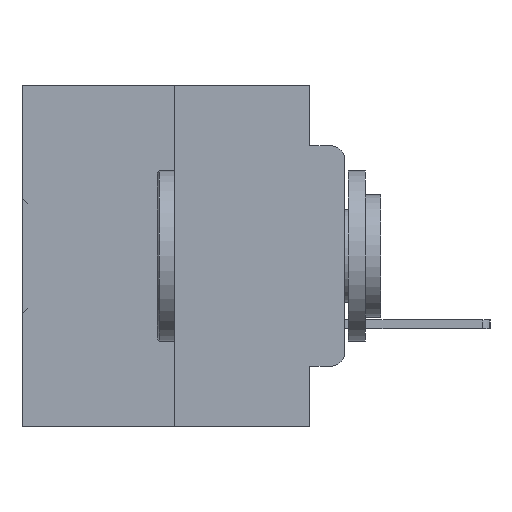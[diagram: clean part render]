
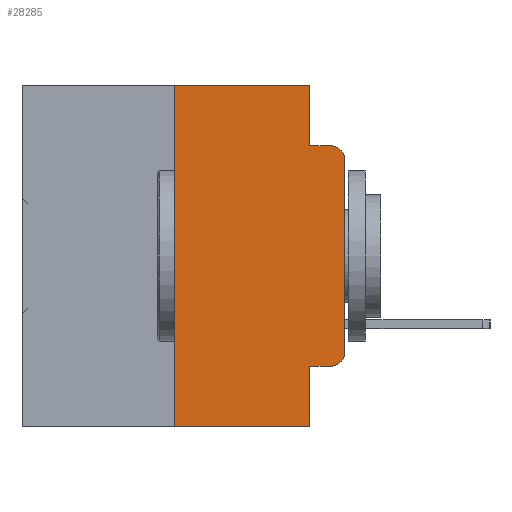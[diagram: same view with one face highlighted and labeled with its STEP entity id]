
A CAD part, left-side view. The second image highlights one B-rep face of the part: STEP entity #28285.
In plain terms, the highlighted planar face has unit normal (-1, 0, 0).
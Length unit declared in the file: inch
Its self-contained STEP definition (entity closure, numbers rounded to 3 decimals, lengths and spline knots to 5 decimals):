
#514 = CIRCLE ( 'NONE', #19929, 0.02 ) ;
#724 = DIRECTION ( 'NONE',  ( 0., 0., -1. ) ) ;
#1535 = LINE ( 'NONE', #25134, #2372 ) ;
#1911 = VECTOR ( 'NONE', #33613, 39.37008 ) ;
#2372 = VECTOR ( 'NONE', #6089, 39.37008 ) ;
#3198 = DIRECTION ( 'NONE',  ( 0., -1., 0. ) ) ;
#3635 = VERTEX_POINT ( 'NONE', #29813 ) ;
#4287 = DIRECTION ( 'NONE',  ( 0., 0., -1. ) ) ;
#4897 = PLANE ( 'NONE',  #5398 ) ;
#5038 = ORIENTED_EDGE ( 'NONE', *, *, #20425, .F. ) ;
#5098 = ORIENTED_EDGE ( 'NONE', *, *, #30010, .F. ) ;
#5297 = ORIENTED_EDGE ( 'NONE', *, *, #9205, .T. ) ;
#5398 = AXIS2_PLACEMENT_3D ( 'NONE', #24024, #26725, #10484 ) ;
#5611 = VERTEX_POINT ( 'NONE', #8649 ) ;
#5665 = EDGE_CURVE ( 'NONE', #26156, #14752, #1535, .T. ) ;
#5706 = FACE_OUTER_BOUND ( 'NONE', #7245, .T. ) ;
#5770 = ORIENTED_EDGE ( 'NONE', *, *, #33626, .T. ) ;
#5880 = VERTEX_POINT ( 'NONE', #28645 ) ;
#6089 = DIRECTION ( 'NONE',  ( 0., 0., 1. ) ) ;
#6663 = CARTESIAN_POINT ( 'NONE',  ( 0., 0.25, 0. ) ) ;
#7099 = ORIENTED_EDGE ( 'NONE', *, *, #5665, .T. ) ;
#7245 = EDGE_LOOP ( 'NONE', ( #7099, #5770, #7549, #5098, #5038, #8175, #5297, #12498, #23703, #16854 ) ) ;
#7288 = CARTESIAN_POINT ( 'NONE',  ( 0., 0.051, 0. ) ) ;
#7549 = ORIENTED_EDGE ( 'NONE', *, *, #31817, .F. ) ;
#8175 = ORIENTED_EDGE ( 'NONE', *, *, #21019, .F. ) ;
#8649 = CARTESIAN_POINT ( 'NONE',  ( 0., 0.051, -0.5 ) ) ;
#8890 = VERTEX_POINT ( 'NONE', #15670 ) ;
#9205 = EDGE_CURVE ( 'NONE', #3635, #5611, #23792, .T. ) ;
#9419 = LINE ( 'NONE', #30806, #1911 ) ;
#9624 = CARTESIAN_POINT ( 'NONE',  ( 0., 0.02, -0.1085 ) ) ;
#10484 = DIRECTION ( 'NONE',  ( 0., 0., -1. ) ) ;
#11902 = EDGE_CURVE ( 'NONE', #12229, #26156, #514, .T. ) ;
#12229 = VERTEX_POINT ( 'NONE', #13226 ) ;
#12356 = DIRECTION ( 'NONE',  ( 0., 0., -1. ) ) ;
#12498 = ORIENTED_EDGE ( 'NONE', *, *, #19168, .F. ) ;
#13226 = CARTESIAN_POINT ( 'NONE',  ( 0., 0.02, -0.4115 ) ) ;
#14493 = LINE ( 'NONE', #26380, #35162 ) ;
#14752 = VERTEX_POINT ( 'NONE', #23008 ) ;
#15238 = CARTESIAN_POINT ( 'NONE',  ( 0., 0., -0.3915 ) ) ;
#15277 = CARTESIAN_POINT ( 'NONE',  ( 0., 0.051, 0. ) ) ;
#15646 = LINE ( 'NONE', #23928, #22023 ) ;
#15670 = CARTESIAN_POINT ( 'NONE',  ( 0., 0.02, -0.0885 ) ) ;
#16402 = LINE ( 'NONE', #23293, #29885 ) ;
#16596 = VECTOR ( 'NONE', #3198, 39.37008 ) ;
#16854 = ORIENTED_EDGE ( 'NONE', *, *, #11902, .T. ) ;
#16970 = CARTESIAN_POINT ( 'NONE',  ( 0., 0.473, -0.5 ) ) ;
#17213 = VECTOR ( 'NONE', #4287, 39.37008 ) ;
#17300 = DIRECTION ( 'NONE',  ( -1., 0., 0. ) ) ;
#17380 = EDGE_CURVE ( 'NONE', #30295, #12229, #9419, .T. ) ;
#18239 = DIRECTION ( 'NONE',  ( 0., -1., 0. ) ) ;
#19168 = EDGE_CURVE ( 'NONE', #30295, #5611, #15646, .T. ) ;
#19306 = VERTEX_POINT ( 'NONE', #32596 ) ;
#19929 = AXIS2_PLACEMENT_3D ( 'NONE', #33432, #17300, #724 ) ;
#20425 = EDGE_CURVE ( 'NONE', #19306, #28181, #16402, .T. ) ;
#21019 = EDGE_CURVE ( 'NONE', #3635, #19306, #29268, .T. ) ;
#22023 = VECTOR ( 'NONE', #32009, 39.37008 ) ;
#23008 = CARTESIAN_POINT ( 'NONE',  ( 0., 0., -0.1085 ) ) ;
#23293 = CARTESIAN_POINT ( 'NONE',  ( 0., 0.473, 0. ) ) ;
#23703 = ORIENTED_EDGE ( 'NONE', *, *, #17380, .T. ) ;
#23792 = LINE ( 'NONE', #16970, #16596 ) ;
#23928 = CARTESIAN_POINT ( 'NONE',  ( 0., 0.051, 0. ) ) ;
#24024 = CARTESIAN_POINT ( 'NONE',  ( 0., 0.473, 0. ) ) ;
#24233 = AXIS2_PLACEMENT_3D ( 'NONE', #9624, #28544, #12356 ) ;
#24727 = CARTESIAN_POINT ( 'NONE',  ( 0., 0.051, -0.4115 ) ) ;
#25134 = CARTESIAN_POINT ( 'NONE',  ( 0., 0., 0. ) ) ;
#25674 = DIRECTION ( 'NONE',  ( 0., 0., 1. ) ) ;
#25984 = DIRECTION ( 'NONE',  ( 0., -1., 0. ) ) ;
#26156 = VERTEX_POINT ( 'NONE', #15238 ) ;
#26380 = CARTESIAN_POINT ( 'NONE',  ( 0., 0.051, -0.0885 ) ) ;
#26725 = DIRECTION ( 'NONE',  ( 1., 0., 0. ) ) ;
#28181 = VERTEX_POINT ( 'NONE', #7288 ) ;
#28285 = ADVANCED_FACE ( 'NONE', ( #5706 ), #4897, .F. ) ;
#28544 = DIRECTION ( 'NONE',  ( -1., 0., 0. ) ) ;
#28645 = CARTESIAN_POINT ( 'NONE',  ( 0., 0.051, -0.0885 ) ) ;
#29268 = LINE ( 'NONE', #6663, #30106 ) ;
#29813 = CARTESIAN_POINT ( 'NONE',  ( 0., 0.25, -0.5 ) ) ;
#29885 = VECTOR ( 'NONE', #25984, 39.37008 ) ;
#30010 = EDGE_CURVE ( 'NONE', #28181, #5880, #31535, .T. ) ;
#30106 = VECTOR ( 'NONE', #25674, 39.37008 ) ;
#30295 = VERTEX_POINT ( 'NONE', #24727 ) ;
#30636 = CIRCLE ( 'NONE', #24233, 0.02 ) ;
#30806 = CARTESIAN_POINT ( 'NONE',  ( 0., 0.051, -0.4115 ) ) ;
#31535 = LINE ( 'NONE', #15277, #17213 ) ;
#31817 = EDGE_CURVE ( 'NONE', #5880, #8890, #14493, .T. ) ;
#32009 = DIRECTION ( 'NONE',  ( 0., 0., -1. ) ) ;
#32596 = CARTESIAN_POINT ( 'NONE',  ( 0., 0.25, 0. ) ) ;
#33432 = CARTESIAN_POINT ( 'NONE',  ( 0., 0.02, -0.3915 ) ) ;
#33613 = DIRECTION ( 'NONE',  ( 0., -1., 0. ) ) ;
#33626 = EDGE_CURVE ( 'NONE', #14752, #8890, #30636, .T. ) ;
#35162 = VECTOR ( 'NONE', #18239, 39.37008 ) ;
